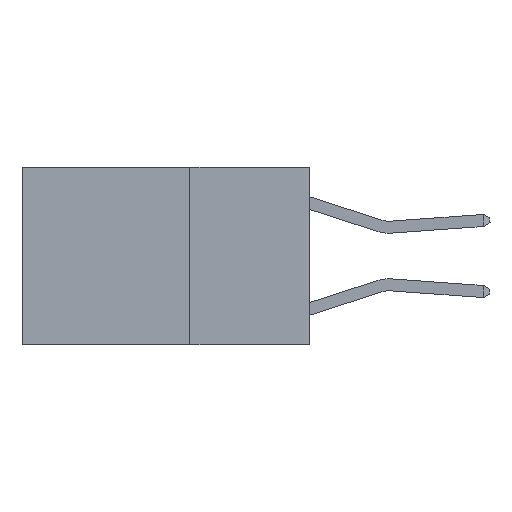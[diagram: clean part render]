
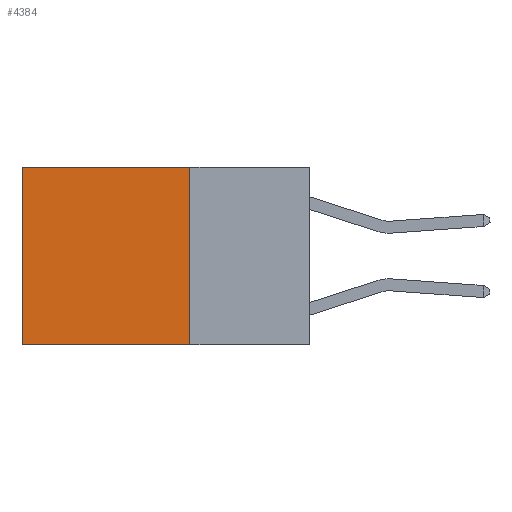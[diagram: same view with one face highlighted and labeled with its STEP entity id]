
A CAD part, left-side view. The second image highlights one B-rep face of the part: STEP entity #4384.
In plain terms, the highlighted planar face has unit normal (-1, 0, 0).
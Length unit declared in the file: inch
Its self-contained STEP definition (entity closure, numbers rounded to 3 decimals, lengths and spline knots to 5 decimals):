
#139 = CARTESIAN_POINT ( 'NONE',  ( 0.2625, 0.25, 0. ) ) ;
#392 = EDGE_CURVE ( 'NONE', #615, #5240, #4431, .T. ) ;
#606 = CARTESIAN_POINT ( 'NONE',  ( 0.2625, 0.25, -0.37 ) ) ;
#615 = VERTEX_POINT ( 'NONE', #5789 ) ;
#688 = EDGE_CURVE ( 'NONE', #8458, #3835, #6379, .T. ) ;
#1110 = DIRECTION ( 'NONE',  ( 0., 1., 0. ) ) ;
#1139 = ORIENTED_EDGE ( 'NONE', *, *, #688, .T. ) ;
#1247 = CARTESIAN_POINT ( 'NONE',  ( 0.2625, 0.6, 0. ) ) ;
#1335 = ORIENTED_EDGE ( 'NONE', *, *, #2215, .F. ) ;
#1631 = ORIENTED_EDGE ( 'NONE', *, *, #392, .F. ) ;
#1816 = ORIENTED_EDGE ( 'NONE', *, *, #2962, .T. ) ;
#2215 = EDGE_CURVE ( 'NONE', #5240, #3835, #2665, .T. ) ;
#2297 = EDGE_LOOP ( 'NONE', ( #1139, #1335, #1631, #1816 ) ) ;
#2665 = LINE ( 'NONE', #606, #6735 ) ;
#2962 = EDGE_CURVE ( 'NONE', #615, #8458, #4882, .T. ) ;
#3312 = PLANE ( 'NONE',  #4813 ) ;
#3450 = DIRECTION ( 'NONE',  ( 0., 1., 0. ) ) ;
#3605 = VECTOR ( 'NONE', #4695, 39.37008 ) ;
#3835 = VERTEX_POINT ( 'NONE', #10192 ) ;
#3858 = FACE_OUTER_BOUND ( 'NONE', #2297, .T. ) ;
#4127 = VECTOR ( 'NONE', #8705, 39.37008 ) ;
#4384 = ADVANCED_FACE ( 'NONE', ( #3858 ), #3312, .F. ) ;
#4431 = LINE ( 'NONE', #10239, #3605 ) ;
#4468 = CARTESIAN_POINT ( 'NONE',  ( 0.2625, 0.25, -0.37 ) ) ;
#4695 = DIRECTION ( 'NONE',  ( 0., 0., -1. ) ) ;
#4813 = AXIS2_PLACEMENT_3D ( 'NONE', #5045, #5087, #10809 ) ;
#4882 = LINE ( 'NONE', #139, #6843 ) ;
#5045 = CARTESIAN_POINT ( 'NONE',  ( 0.2625, 0.25, 0. ) ) ;
#5087 = DIRECTION ( 'NONE',  ( 1., 0., 0. ) ) ;
#5240 = VERTEX_POINT ( 'NONE', #4468 ) ;
#5789 = CARTESIAN_POINT ( 'NONE',  ( 0.2625, 0.25, 0. ) ) ;
#6379 = LINE ( 'NONE', #1247, #4127 ) ;
#6735 = VECTOR ( 'NONE', #3450, 39.37008 ) ;
#6843 = VECTOR ( 'NONE', #1110, 39.37008 ) ;
#7678 = CARTESIAN_POINT ( 'NONE',  ( 0.2625, 0.6, 0. ) ) ;
#8458 = VERTEX_POINT ( 'NONE', #7678 ) ;
#8705 = DIRECTION ( 'NONE',  ( 0., 0., -1. ) ) ;
#10192 = CARTESIAN_POINT ( 'NONE',  ( 0.2625, 0.6, -0.37 ) ) ;
#10239 = CARTESIAN_POINT ( 'NONE',  ( 0.2625, 0.25, 0. ) ) ;
#10809 = DIRECTION ( 'NONE',  ( 0., 0., -1. ) ) ;
